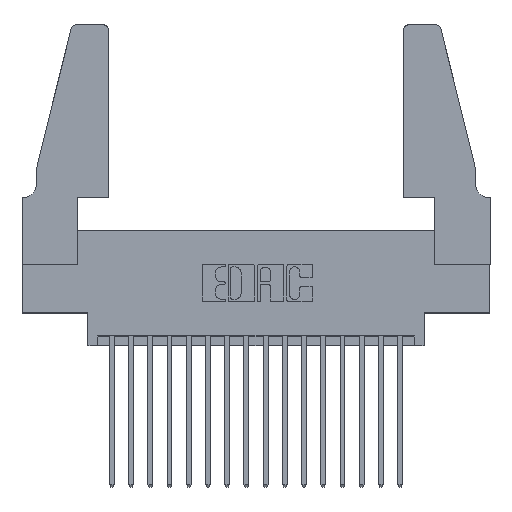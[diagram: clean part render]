
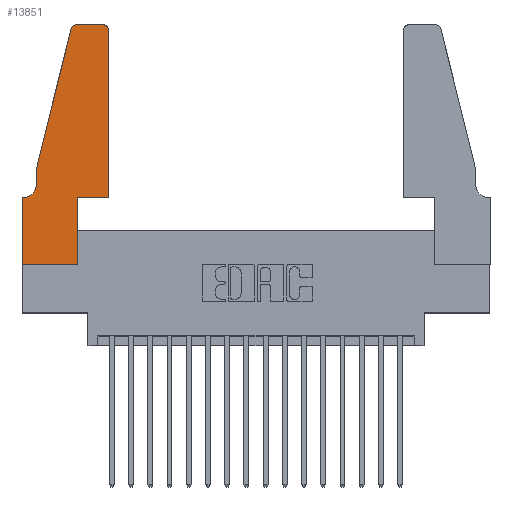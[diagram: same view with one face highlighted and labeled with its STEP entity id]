
A CAD part, top view. The second image highlights one B-rep face of the part: STEP entity #13851.
In plain terms, the highlighted planar face has unit normal (0, 0, 1).
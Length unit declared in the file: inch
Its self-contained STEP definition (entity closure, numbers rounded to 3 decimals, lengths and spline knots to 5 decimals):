
#19 = EDGE_CURVE ( 'NONE', #17987, #3476, #13435, .T. ) ;
#22 = CARTESIAN_POINT ( 'NONE',  ( 0.4505, 0.35, 0.37 ) ) ;
#63 = VERTEX_POINT ( 'NONE', #7761 ) ;
#75 = VERTEX_POINT ( 'NONE', #14849 ) ;
#191 = EDGE_CURVE ( 'NONE', #7866, #17987, #8530, .T. ) ;
#256 = VECTOR ( 'NONE', #855, 39.37008 ) ;
#600 = LINE ( 'NONE', #1179, #2836 ) ;
#707 = VECTOR ( 'NONE', #7932, 39.37008 ) ;
#773 = ORIENTED_EDGE ( 'NONE', *, *, #18104, .T. ) ;
#855 = DIRECTION ( 'NONE',  ( -0.239, -0.971, 0. ) ) ;
#896 = CARTESIAN_POINT ( 'NONE',  ( 0., 0., 0.37 ) ) ;
#1062 = AXIS2_PLACEMENT_3D ( 'NONE', #9065, #10432, #14689 ) ;
#1179 = CARTESIAN_POINT ( 'NONE',  ( 0.4505, 0.35, 0.37 ) ) ;
#1284 = CARTESIAN_POINT ( 'NONE',  ( 0.2865, 0., 0.37 ) ) ;
#1433 = DIRECTION ( 'NONE',  ( 0., 1., 0. ) ) ;
#1533 = VERTEX_POINT ( 'NONE', #8898 ) ;
#1710 = VECTOR ( 'NONE', #16270, 39.37008 ) ;
#1982 = CARTESIAN_POINT ( 'NONE',  ( 0.0755, 0.35, 0.37 ) ) ;
#2154 = DIRECTION ( 'NONE',  ( 1., 0., 0. ) ) ;
#2334 = CIRCLE ( 'NONE', #7868, 0.07 ) ;
#2585 = VERTEX_POINT ( 'NONE', #22 ) ;
#2836 = VECTOR ( 'NONE', #1433, 39.37008 ) ;
#2921 = CARTESIAN_POINT ( 'NONE',  ( 0., 0., 0.37 ) ) ;
#3235 = VERTEX_POINT ( 'NONE', #7137 ) ;
#3476 = VERTEX_POINT ( 'NONE', #6133 ) ;
#3685 = DIRECTION ( 'NONE',  ( 1., 0., 0. ) ) ;
#3935 = VECTOR ( 'NONE', #16860, 39.37008 ) ;
#4095 = ORIENTED_EDGE ( 'NONE', *, *, #19, .T. ) ;
#4274 = CARTESIAN_POINT ( 'NONE',  ( 0.4505, 0.35, 0.37 ) ) ;
#4620 = EDGE_CURVE ( 'NONE', #3476, #7177, #18004, .T. ) ;
#5245 = LINE ( 'NONE', #5721, #14137 ) ;
#5427 = CARTESIAN_POINT ( 'NONE',  ( 0.284, 1.22, 0.37 ) ) ;
#5575 = EDGE_CURVE ( 'NONE', #9525, #17394, #12818, .T. ) ;
#5721 = CARTESIAN_POINT ( 'NONE',  ( 0.0755, 0.5, 0.37 ) ) ;
#5909 = DIRECTION ( 'NONE',  ( 1., 0., 0. ) ) ;
#5995 = DIRECTION ( 'NONE',  ( -1., 0., 0. ) ) ;
#6133 = CARTESIAN_POINT ( 'NONE',  ( 0.25487, 1.22718, 0.37 ) ) ;
#6179 = DIRECTION ( 'NONE',  ( 1., 0., 0. ) ) ;
#6287 = CARTESIAN_POINT ( 'NONE',  ( 0.2605, 1.25, 0.37 ) ) ;
#6447 = AXIS2_PLACEMENT_3D ( 'NONE', #7863, #9170, #2154 ) ;
#6449 = EDGE_CURVE ( 'NONE', #3235, #2585, #13723, .T. ) ;
#7037 = ORIENTED_EDGE ( 'NONE', *, *, #17648, .T. ) ;
#7077 = VECTOR ( 'NONE', #5909, 39.37008 ) ;
#7119 = DIRECTION ( 'NONE',  ( 0., -1., 0. ) ) ;
#7137 = CARTESIAN_POINT ( 'NONE',  ( 0.2865, 0.35, 0.37 ) ) ;
#7177 = VERTEX_POINT ( 'NONE', #18019 ) ;
#7317 = LINE ( 'NONE', #12269, #707 ) ;
#7330 = ORIENTED_EDGE ( 'NONE', *, *, #16433, .T. ) ;
#7761 = CARTESIAN_POINT ( 'NONE',  ( 0., 0.35, 0.37 ) ) ;
#7863 = CARTESIAN_POINT ( 'NONE',  ( 0., 0.35, 0.37 ) ) ;
#7866 = VERTEX_POINT ( 'NONE', #13553 ) ;
#7868 = AXIS2_PLACEMENT_3D ( 'NONE', #12177, #17688, #7965 ) ;
#7932 = DIRECTION ( 'NONE',  ( 0., 1., 0. ) ) ;
#7965 = DIRECTION ( 'NONE',  ( -1., 0., 0. ) ) ;
#8024 = CARTESIAN_POINT ( 'NONE',  ( 0.284, 1.25, 0.37 ) ) ;
#8530 = LINE ( 'NONE', #6287, #1710 ) ;
#8898 = CARTESIAN_POINT ( 'NONE',  ( 0.4505, 1.22, 0.37 ) ) ;
#8969 = LINE ( 'NONE', #1982, #9422 ) ;
#9065 = CARTESIAN_POINT ( 'NONE',  ( 0.4205, 1.22, 0.37 ) ) ;
#9170 = DIRECTION ( 'NONE',  ( 0., 0., 1. ) ) ;
#9422 = VECTOR ( 'NONE', #5995, 39.37008 ) ;
#9423 = CARTESIAN_POINT ( 'NONE',  ( 0.0755, 0.5, 0.37 ) ) ;
#9525 = VERTEX_POINT ( 'NONE', #10425 ) ;
#9911 = EDGE_CURVE ( 'NONE', #1533, #7866, #18051, .T. ) ;
#10067 = AXIS2_PLACEMENT_3D ( 'NONE', #5427, #12970, #6179 ) ;
#10425 = CARTESIAN_POINT ( 'NONE',  ( 0., 0., 0.37 ) ) ;
#10432 = DIRECTION ( 'NONE',  ( 0., 0., 1. ) ) ;
#10906 = ORIENTED_EDGE ( 'NONE', *, *, #15416, .T. ) ;
#11133 = ORIENTED_EDGE ( 'NONE', *, *, #5575, .T. ) ;
#11457 = VERTEX_POINT ( 'NONE', #16450 ) ;
#11509 = EDGE_LOOP ( 'NONE', ( #11659, #4095, #11524, #7037, #7330, #17612, #773, #11133, #17240, #14173, #10906, #15131 ) ) ;
#11524 = ORIENTED_EDGE ( 'NONE', *, *, #4620, .T. ) ;
#11659 = ORIENTED_EDGE ( 'NONE', *, *, #191, .T. ) ;
#12177 = CARTESIAN_POINT ( 'NONE',  ( 0.0055, 0.42, 0.37 ) ) ;
#12269 = CARTESIAN_POINT ( 'NONE',  ( 0.2865, 0.35, 0.37 ) ) ;
#12524 = EDGE_CURVE ( 'NONE', #17394, #3235, #7317, .T. ) ;
#12818 = LINE ( 'NONE', #896, #13715 ) ;
#12970 = DIRECTION ( 'NONE',  ( 0., 0., 1. ) ) ;
#13435 = CIRCLE ( 'NONE', #10067, 0.03 ) ;
#13553 = CARTESIAN_POINT ( 'NONE',  ( 0.4205, 1.25, 0.37 ) ) ;
#13645 = LINE ( 'NONE', #2921, #3935 ) ;
#13715 = VECTOR ( 'NONE', #3685, 39.37008 ) ;
#13723 = LINE ( 'NONE', #4274, #7077 ) ;
#13851 = ADVANCED_FACE ( 'NONE', ( #17732 ), #15098, .T. ) ;
#14137 = VECTOR ( 'NONE', #7119, 39.37008 ) ;
#14173 = ORIENTED_EDGE ( 'NONE', *, *, #6449, .T. ) ;
#14689 = DIRECTION ( 'NONE',  ( 1., 0., 0. ) ) ;
#14849 = CARTESIAN_POINT ( 'NONE',  ( 0.0055, 0.35, 0.37 ) ) ;
#15098 = PLANE ( 'NONE',  #6447 ) ;
#15131 = ORIENTED_EDGE ( 'NONE', *, *, #9911, .T. ) ;
#15416 = EDGE_CURVE ( 'NONE', #2585, #1533, #600, .T. ) ;
#15640 = EDGE_CURVE ( 'NONE', #75, #63, #8969, .T. ) ;
#16270 = DIRECTION ( 'NONE',  ( -1., 0., 0. ) ) ;
#16433 = EDGE_CURVE ( 'NONE', #11457, #75, #2334, .T. ) ;
#16450 = CARTESIAN_POINT ( 'NONE',  ( 0.0755, 0.42, 0.37 ) ) ;
#16860 = DIRECTION ( 'NONE',  ( 0., -1., 0. ) ) ;
#17240 = ORIENTED_EDGE ( 'NONE', *, *, #12524, .T. ) ;
#17394 = VERTEX_POINT ( 'NONE', #1284 ) ;
#17612 = ORIENTED_EDGE ( 'NONE', *, *, #15640, .T. ) ;
#17648 = EDGE_CURVE ( 'NONE', #7177, #11457, #5245, .T. ) ;
#17688 = DIRECTION ( 'NONE',  ( 0., 0., -1. ) ) ;
#17732 = FACE_OUTER_BOUND ( 'NONE', #11509, .T. ) ;
#17987 = VERTEX_POINT ( 'NONE', #8024 ) ;
#18004 = LINE ( 'NONE', #9423, #256 ) ;
#18019 = CARTESIAN_POINT ( 'NONE',  ( 0.0755, 0.5, 0.37 ) ) ;
#18051 = CIRCLE ( 'NONE', #1062, 0.03 ) ;
#18104 = EDGE_CURVE ( 'NONE', #63, #9525, #13645, .T. ) ;
